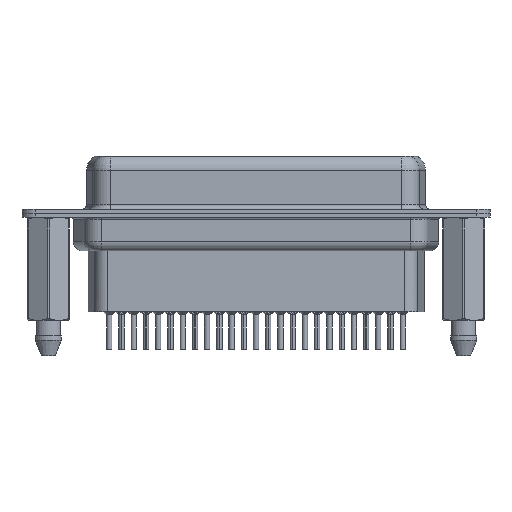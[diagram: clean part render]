
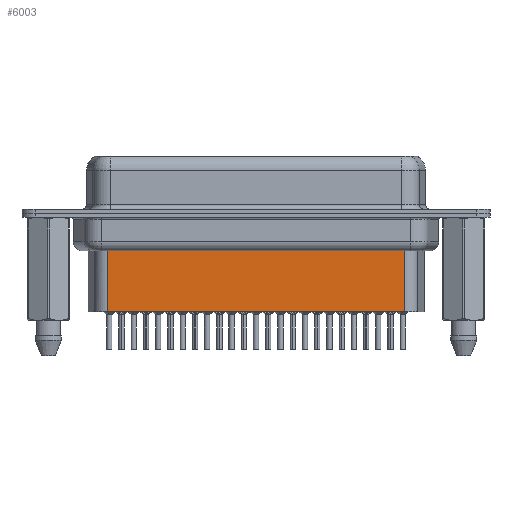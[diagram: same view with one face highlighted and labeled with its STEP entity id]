
A CAD part, front view. The second image highlights one B-rep face of the part: STEP entity #6003.
In plain terms, the highlighted planar face has unit normal (0, -1, 0).
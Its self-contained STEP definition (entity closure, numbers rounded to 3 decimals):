
#244 = VERTEX_POINT ( 'NONE', #20845 ) ;
#460 = VERTEX_POINT ( 'NONE', #5986 ) ;
#840 = ORIENTED_EDGE ( 'NONE', *, *, #20978, .F. ) ;
#1782 = CARTESIAN_POINT ( 'NONE',  ( 40.344, -3.5, -4.097 ) ) ;
#2858 = DIRECTION ( 'NONE',  ( 1., 0., 0. ) ) ;
#4222 = EDGE_LOOP ( 'NONE', ( #840, #13251, #23294, #22897 ) ) ;
#5986 = CARTESIAN_POINT ( 'NONE',  ( 40.344, -3.5, -11.15 ) ) ;
#6003 = ADVANCED_FACE ( 'NONE', ( #24790 ), #20341, .T. ) ;
#6521 = DIRECTION ( 'NONE',  ( -1., 0., 0. ) ) ;
#6744 = DIRECTION ( 'NONE',  ( -1., 0., 0. ) ) ;
#6860 = VERTEX_POINT ( 'NONE', #1782 ) ;
#8600 = CARTESIAN_POINT ( 'NONE',  ( 6.706, -3.5, -11.15 ) ) ;
#9401 = AXIS2_PLACEMENT_3D ( 'NONE', #22992, #13735, #2858 ) ;
#12911 = EDGE_CURVE ( 'NONE', #13323, #244, #26019, .T. ) ;
#13251 = ORIENTED_EDGE ( 'NONE', *, *, #16251, .T. ) ;
#13323 = VERTEX_POINT ( 'NONE', #23229 ) ;
#13735 = DIRECTION ( 'NONE',  ( 0., -1., 0. ) ) ;
#13799 = LINE ( 'NONE', #17923, #17053 ) ;
#15180 = VECTOR ( 'NONE', #6521, 1000. ) ;
#15303 = VECTOR ( 'NONE', #28515, 1000. ) ;
#16251 = EDGE_CURVE ( 'NONE', #6860, #13323, #13799, .T. ) ;
#17053 = VECTOR ( 'NONE', #6744, 1000. ) ;
#17121 = EDGE_CURVE ( 'NONE', #460, #244, #19748, .T. ) ;
#17310 = CARTESIAN_POINT ( 'NONE',  ( 40.344, -3.5, -3.1 ) ) ;
#17923 = CARTESIAN_POINT ( 'NONE',  ( 6.459, -3.5, -4.097 ) ) ;
#19748 = LINE ( 'NONE', #8600, #15180 ) ;
#20341 = PLANE ( 'NONE',  #9401 ) ;
#20845 = CARTESIAN_POINT ( 'NONE',  ( 6.706, -3.5, -11.15 ) ) ;
#20978 = EDGE_CURVE ( 'NONE', #6860, #460, #26584, .T. ) ;
#21564 = DIRECTION ( 'NONE',  ( 0., 0., -1. ) ) ;
#22897 = ORIENTED_EDGE ( 'NONE', *, *, #17121, .F. ) ;
#22992 = CARTESIAN_POINT ( 'NONE',  ( 6.706, -3.5, -3.1 ) ) ;
#23229 = CARTESIAN_POINT ( 'NONE',  ( 6.706, -3.5, -4.097 ) ) ;
#23294 = ORIENTED_EDGE ( 'NONE', *, *, #12911, .T. ) ;
#23791 = CARTESIAN_POINT ( 'NONE',  ( 6.706, -3.5, -3.1 ) ) ;
#24790 = FACE_OUTER_BOUND ( 'NONE', #4222, .T. ) ;
#26019 = LINE ( 'NONE', #23791, #26474 ) ;
#26474 = VECTOR ( 'NONE', #21564, 1000. ) ;
#26584 = LINE ( 'NONE', #17310, #15303 ) ;
#28515 = DIRECTION ( 'NONE',  ( 0., 0., -1. ) ) ;
